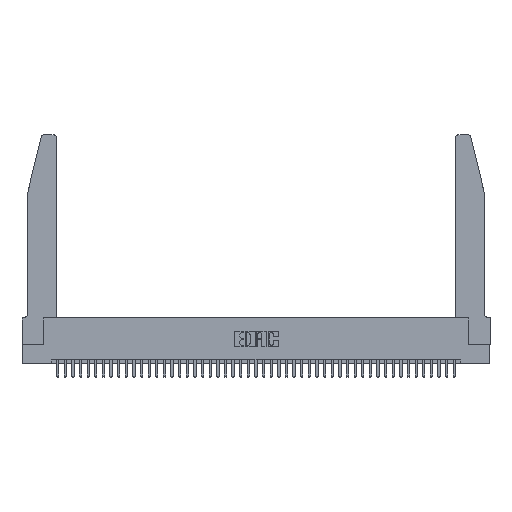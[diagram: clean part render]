
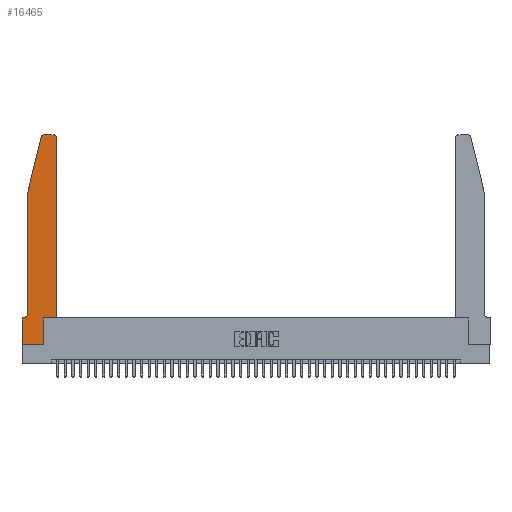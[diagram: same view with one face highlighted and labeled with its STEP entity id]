
A CAD part, top view. The second image highlights one B-rep face of the part: STEP entity #16465.
In plain terms, the highlighted planar face has unit normal (0, 0, 1).
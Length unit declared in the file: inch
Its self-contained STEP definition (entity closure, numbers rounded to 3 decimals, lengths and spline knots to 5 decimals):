
#1037 = VECTOR ( 'NONE', #31099, 39.37008 ) ;
#2525 = VECTOR ( 'NONE', #19007, 39.37008 ) ;
#2883 = CARTESIAN_POINT ( 'NONE',  ( 0.4205, 2.75, 0.37 ) ) ;
#3073 = VERTEX_POINT ( 'NONE', #3683 ) ;
#3259 = CARTESIAN_POINT ( 'NONE',  ( 0.0755, 0.35, 0.37 ) ) ;
#3279 = AXIS2_PLACEMENT_3D ( 'NONE', #37198, #16537, #40680 ) ;
#3683 = CARTESIAN_POINT ( 'NONE',  ( 0.25487, 2.72718, 0.37 ) ) ;
#4298 = PLANE ( 'NONE',  #14021 ) ;
#4918 = VECTOR ( 'NONE', #35976, 39.37008 ) ;
#5284 = VERTEX_POINT ( 'NONE', #43086 ) ;
#5490 = LINE ( 'NONE', #16358, #15898 ) ;
#6391 = VERTEX_POINT ( 'NONE', #14837 ) ;
#6685 = CARTESIAN_POINT ( 'NONE',  ( 0.2605, 2.75, 0.37 ) ) ;
#6759 = CARTESIAN_POINT ( 'NONE',  ( 0.4505, 2.72, 0.37 ) ) ;
#6811 = DIRECTION ( 'NONE',  ( -1., 0., 0. ) ) ;
#7293 = CARTESIAN_POINT ( 'NONE',  ( 0.2865, 0.35, 0.37 ) ) ;
#7901 = CARTESIAN_POINT ( 'NONE',  ( 0.0755, 0.42, 0.37 ) ) ;
#7909 = EDGE_CURVE ( 'NONE', #21782, #39054, #33862, .T. ) ;
#8661 = VERTEX_POINT ( 'NONE', #7293 ) ;
#9944 = CARTESIAN_POINT ( 'NONE',  ( 0.4505, 0.35, 0.37 ) ) ;
#10201 = DIRECTION ( 'NONE',  ( -1., 0., 0. ) ) ;
#10701 = ORIENTED_EDGE ( 'NONE', *, *, #36453, .T. ) ;
#10993 = CARTESIAN_POINT ( 'NONE',  ( 0.2865, 0., 0.37 ) ) ;
#11945 = ORIENTED_EDGE ( 'NONE', *, *, #18207, .T. ) ;
#12176 = CARTESIAN_POINT ( 'NONE',  ( 0., 0., 0.37 ) ) ;
#13097 = ORIENTED_EDGE ( 'NONE', *, *, #35382, .T. ) ;
#13123 = ORIENTED_EDGE ( 'NONE', *, *, #26974, .T. ) ;
#13471 = DIRECTION ( 'NONE',  ( 1., 0., 0. ) ) ;
#13926 = EDGE_CURVE ( 'NONE', #6391, #43629, #21102, .T. ) ;
#13937 = CARTESIAN_POINT ( 'NONE',  ( 0.0755, 2., 0.37 ) ) ;
#14021 = AXIS2_PLACEMENT_3D ( 'NONE', #35541, #14902, #39049 ) ;
#14208 = CARTESIAN_POINT ( 'NONE',  ( 0.0055, 0.42, 0.37 ) ) ;
#14837 = CARTESIAN_POINT ( 'NONE',  ( 0., 0.35, 0.37 ) ) ;
#14902 = DIRECTION ( 'NONE',  ( 0., 0., 1. ) ) ;
#15038 = VECTOR ( 'NONE', #6811, 39.37008 ) ;
#15335 = CARTESIAN_POINT ( 'NONE',  ( 0.4505, 0.35, 0.37 ) ) ;
#15898 = VECTOR ( 'NONE', #19820, 39.37008 ) ;
#16332 = LINE ( 'NONE', #12176, #32457 ) ;
#16358 = CARTESIAN_POINT ( 'NONE',  ( 0.2865, 0.35, 0.37 ) ) ;
#16465 = ADVANCED_FACE ( 'NONE', ( #43056 ), #4298, .T. ) ;
#16537 = DIRECTION ( 'NONE',  ( 0., 0., 1. ) ) ;
#16853 = LINE ( 'NONE', #6685, #23827 ) ;
#17677 = DIRECTION ( 'NONE',  ( -1., 0., 0. ) ) ;
#17894 = VERTEX_POINT ( 'NONE', #32603 ) ;
#18096 = EDGE_CURVE ( 'NONE', #22474, #8661, #5490, .T. ) ;
#18207 = EDGE_CURVE ( 'NONE', #17894, #39936, #20741, .T. ) ;
#18628 = CARTESIAN_POINT ( 'NONE',  ( 0.284, 2.72, 0.37 ) ) ;
#18707 = CIRCLE ( 'NONE', #22057, 0.07 ) ;
#19007 = DIRECTION ( 'NONE',  ( 0., -1., 0. ) ) ;
#19023 = DIRECTION ( 'NONE',  ( -0.239, -0.971, 0. ) ) ;
#19354 = LINE ( 'NONE', #9944, #27400 ) ;
#19820 = DIRECTION ( 'NONE',  ( 0., 1., 0. ) ) ;
#20741 = LINE ( 'NONE', #13937, #1037 ) ;
#20900 = CIRCLE ( 'NONE', #44622, 0.03 ) ;
#21102 = LINE ( 'NONE', #36195, #2525 ) ;
#21782 = VERTEX_POINT ( 'NONE', #6759 ) ;
#22057 = AXIS2_PLACEMENT_3D ( 'NONE', #14208, #38366, #17677 ) ;
#22080 = DIRECTION ( 'NONE',  ( 1., 0., 0. ) ) ;
#22317 = CARTESIAN_POINT ( 'NONE',  ( 0.0755, 2., 0.37 ) ) ;
#22474 = VERTEX_POINT ( 'NONE', #10993 ) ;
#22576 = DIRECTION ( 'NONE',  ( 1., 0., 0. ) ) ;
#23523 = ORIENTED_EDGE ( 'NONE', *, *, #30913, .T. ) ;
#23827 = VECTOR ( 'NONE', #10201, 39.37008 ) ;
#25322 = ORIENTED_EDGE ( 'NONE', *, *, #38465, .T. ) ;
#26974 = EDGE_CURVE ( 'NONE', #42456, #3073, #20900, .T. ) ;
#27039 = ORIENTED_EDGE ( 'NONE', *, *, #27741, .T. ) ;
#27252 = LINE ( 'NONE', #22317, #34291 ) ;
#27400 = VECTOR ( 'NONE', #13471, 39.37008 ) ;
#27407 = ORIENTED_EDGE ( 'NONE', *, *, #7909, .T. ) ;
#27461 = EDGE_CURVE ( 'NONE', #39936, #28197, #18707, .T. ) ;
#27741 = EDGE_CURVE ( 'NONE', #3073, #17894, #27252, .T. ) ;
#28197 = VERTEX_POINT ( 'NONE', #32047 ) ;
#30913 = EDGE_CURVE ( 'NONE', #43629, #22474, #16332, .T. ) ;
#31099 = DIRECTION ( 'NONE',  ( 0., -1., 0. ) ) ;
#31474 = LINE ( 'NONE', #15335, #4918 ) ;
#31717 = CARTESIAN_POINT ( 'NONE',  ( 0., 0., 0.37 ) ) ;
#31807 = CARTESIAN_POINT ( 'NONE',  ( 0.284, 2.75, 0.37 ) ) ;
#32047 = CARTESIAN_POINT ( 'NONE',  ( 0.0055, 0.35, 0.37 ) ) ;
#32373 = EDGE_LOOP ( 'NONE', ( #10701, #13123, #27039, #11945, #44409, #25322, #37208, #23523, #41192, #34329, #13097, #27407 ) ) ;
#32457 = VECTOR ( 'NONE', #22576, 39.37008 ) ;
#32603 = CARTESIAN_POINT ( 'NONE',  ( 0.0755, 2., 0.37 ) ) ;
#33112 = EDGE_CURVE ( 'NONE', #8661, #5284, #19354, .T. ) ;
#33862 = CIRCLE ( 'NONE', #3279, 0.03 ) ;
#34291 = VECTOR ( 'NONE', #19023, 39.37008 ) ;
#34329 = ORIENTED_EDGE ( 'NONE', *, *, #33112, .T. ) ;
#35382 = EDGE_CURVE ( 'NONE', #5284, #21782, #31474, .T. ) ;
#35541 = CARTESIAN_POINT ( 'NONE',  ( 0., 0.35, 0.37 ) ) ;
#35976 = DIRECTION ( 'NONE',  ( 0., 1., 0. ) ) ;
#36195 = CARTESIAN_POINT ( 'NONE',  ( 0., 0., 0.37 ) ) ;
#36453 = EDGE_CURVE ( 'NONE', #39054, #42456, #16853, .T. ) ;
#37198 = CARTESIAN_POINT ( 'NONE',  ( 0.4205, 2.72, 0.37 ) ) ;
#37208 = ORIENTED_EDGE ( 'NONE', *, *, #13926, .T. ) ;
#38366 = DIRECTION ( 'NONE',  ( 0., 0., -1. ) ) ;
#38465 = EDGE_CURVE ( 'NONE', #28197, #6391, #42581, .T. ) ;
#39049 = DIRECTION ( 'NONE',  ( 1., 0., 0. ) ) ;
#39054 = VERTEX_POINT ( 'NONE', #2883 ) ;
#39936 = VERTEX_POINT ( 'NONE', #7901 ) ;
#40680 = DIRECTION ( 'NONE',  ( 1., 0., 0. ) ) ;
#41192 = ORIENTED_EDGE ( 'NONE', *, *, #18096, .T. ) ;
#42456 = VERTEX_POINT ( 'NONE', #31807 ) ;
#42581 = LINE ( 'NONE', #3259, #15038 ) ;
#42776 = DIRECTION ( 'NONE',  ( 0., 0., 1. ) ) ;
#43056 = FACE_OUTER_BOUND ( 'NONE', #32373, .T. ) ;
#43086 = CARTESIAN_POINT ( 'NONE',  ( 0.4505, 0.35, 0.37 ) ) ;
#43629 = VERTEX_POINT ( 'NONE', #31717 ) ;
#44409 = ORIENTED_EDGE ( 'NONE', *, *, #27461, .T. ) ;
#44622 = AXIS2_PLACEMENT_3D ( 'NONE', #18628, #42776, #22080 ) ;
